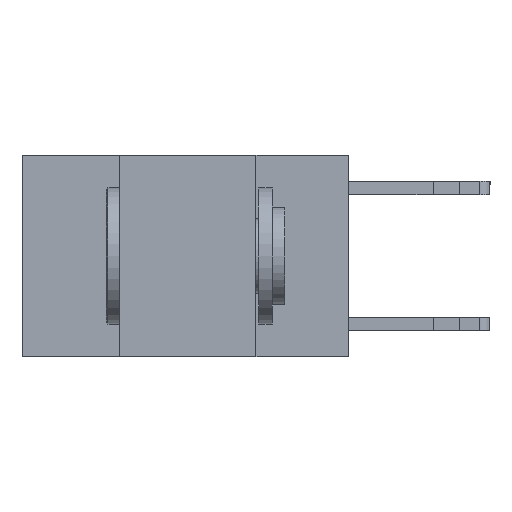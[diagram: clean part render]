
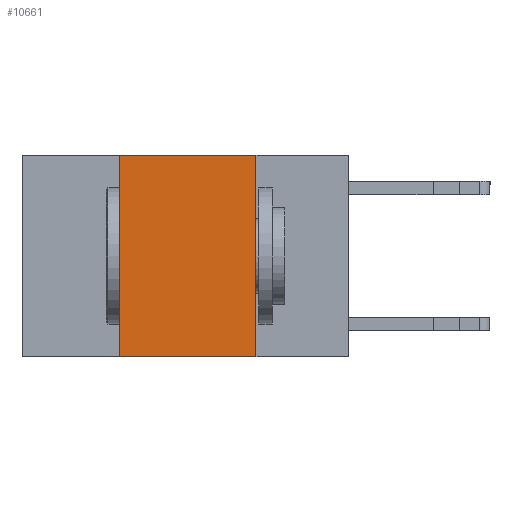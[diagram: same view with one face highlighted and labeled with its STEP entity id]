
A CAD part, left-side view. The second image highlights one B-rep face of the part: STEP entity #10661.
In plain terms, the highlighted planar face has unit normal (-1, 0, 0).
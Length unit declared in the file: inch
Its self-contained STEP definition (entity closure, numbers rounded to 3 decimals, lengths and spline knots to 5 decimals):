
#508 = VERTEX_POINT ( 'NONE', #9239 ) ;
#768 = DIRECTION ( 'NONE',  ( 0., 0., -1. ) ) ;
#1568 = CARTESIAN_POINT ( 'NONE',  ( 0., 0.17, -0.37 ) ) ;
#3231 = ORIENTED_EDGE ( 'NONE', *, *, #12674, .F. ) ;
#3592 = DIRECTION ( 'NONE',  ( 0., -1., 0. ) ) ;
#5314 = DIRECTION ( 'NONE',  ( 0., 0., 1. ) ) ;
#5500 = CARTESIAN_POINT ( 'NONE',  ( 0., 0.6, 0. ) ) ;
#5549 = VECTOR ( 'NONE', #768, 39.37008 ) ;
#6319 = CARTESIAN_POINT ( 'NONE',  ( 0., 0.6, 0. ) ) ;
#6322 = VERTEX_POINT ( 'NONE', #13355 ) ;
#8559 = LINE ( 'NONE', #21436, #5549 ) ;
#9239 = CARTESIAN_POINT ( 'NONE',  ( 0., 0.42, 0. ) ) ;
#9612 = ORIENTED_EDGE ( 'NONE', *, *, #20762, .F. ) ;
#9792 = EDGE_CURVE ( 'NONE', #18877, #11173, #11767, .T. ) ;
#10661 = ADVANCED_FACE ( 'NONE', ( #23508 ), #23002, .F. ) ;
#10954 = EDGE_LOOP ( 'NONE', ( #13373, #9612, #3231, #22735 ) ) ;
#11173 = VERTEX_POINT ( 'NONE', #1568 ) ;
#11767 = LINE ( 'NONE', #13842, #14986 ) ;
#12450 = VECTOR ( 'NONE', #5314, 39.37008 ) ;
#12674 = EDGE_CURVE ( 'NONE', #18877, #508, #20296, .T. ) ;
#13355 = CARTESIAN_POINT ( 'NONE',  ( 0., 0.17, 0. ) ) ;
#13373 = ORIENTED_EDGE ( 'NONE', *, *, #22065, .F. ) ;
#13842 = CARTESIAN_POINT ( 'NONE',  ( 0., 0.6, -0.37 ) ) ;
#14986 = VECTOR ( 'NONE', #21019, 39.37008 ) ;
#16679 = VECTOR ( 'NONE', #3592, 39.37008 ) ;
#17803 = DIRECTION ( 'NONE',  ( 0., 0., -1. ) ) ;
#18318 = LINE ( 'NONE', #5500, #16679 ) ;
#18877 = VERTEX_POINT ( 'NONE', #21965 ) ;
#19748 = DIRECTION ( 'NONE',  ( 1., 0., 0. ) ) ;
#20296 = LINE ( 'NONE', #21989, #12450 ) ;
#20762 = EDGE_CURVE ( 'NONE', #508, #6322, #18318, .T. ) ;
#21019 = DIRECTION ( 'NONE',  ( 0., -1., 0. ) ) ;
#21120 = AXIS2_PLACEMENT_3D ( 'NONE', #6319, #19748, #17803 ) ;
#21436 = CARTESIAN_POINT ( 'NONE',  ( 0., 0.17, 0. ) ) ;
#21965 = CARTESIAN_POINT ( 'NONE',  ( 0., 0.42, -0.37 ) ) ;
#21989 = CARTESIAN_POINT ( 'NONE',  ( 0., 0.42, 0. ) ) ;
#22065 = EDGE_CURVE ( 'NONE', #6322, #11173, #8559, .T. ) ;
#22735 = ORIENTED_EDGE ( 'NONE', *, *, #9792, .T. ) ;
#23002 = PLANE ( 'NONE',  #21120 ) ;
#23508 = FACE_OUTER_BOUND ( 'NONE', #10954, .T. ) ;
